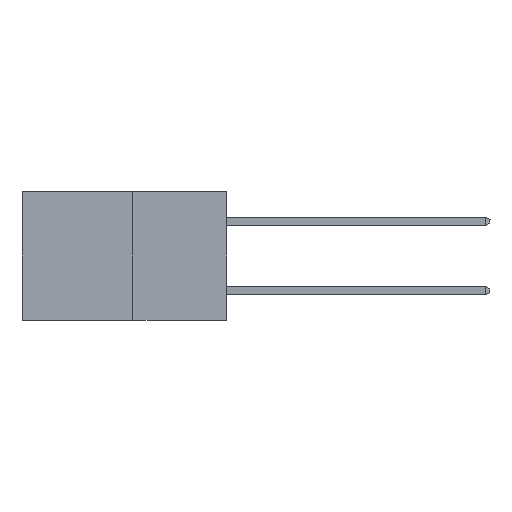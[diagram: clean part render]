
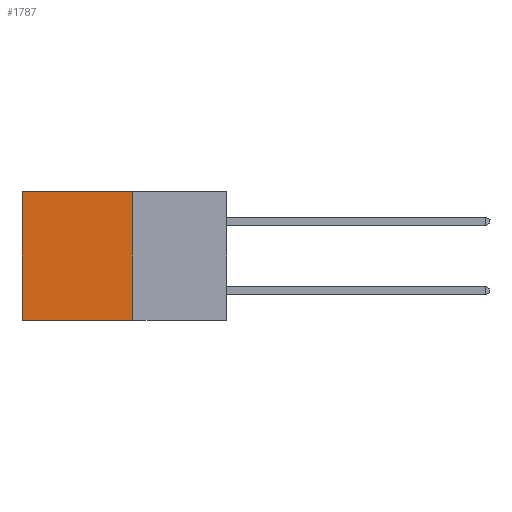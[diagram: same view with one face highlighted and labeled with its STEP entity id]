
A CAD part, left-side view. The second image highlights one B-rep face of the part: STEP entity #1787.
In plain terms, the highlighted planar face has unit normal (-1, 0, 0).
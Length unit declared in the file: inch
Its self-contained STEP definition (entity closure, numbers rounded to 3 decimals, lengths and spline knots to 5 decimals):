
#195 = VECTOR ( 'NONE', #348, 39.37008 ) ;
#211 = FACE_OUTER_BOUND ( 'NONE', #3395, .T. ) ;
#271 = DIRECTION ( 'NONE',  ( 0., 1., 0. ) ) ;
#348 = DIRECTION ( 'NONE',  ( 0., 0., -1. ) ) ;
#1368 = EDGE_CURVE ( 'NONE', #9910, #1708, #5854, .T. ) ;
#1708 = VERTEX_POINT ( 'NONE', #13616 ) ;
#1787 = ADVANCED_FACE ( 'NONE', ( #211 ), #13974, .F. ) ;
#1894 = CARTESIAN_POINT ( 'NONE',  ( 0.277, 0.27, -0.37 ) ) ;
#2162 = EDGE_CURVE ( 'NONE', #2884, #9910, #3405, .T. ) ;
#2731 = CARTESIAN_POINT ( 'NONE',  ( 0.277, 0.27, -0.37 ) ) ;
#2884 = VERTEX_POINT ( 'NONE', #9032 ) ;
#3395 = EDGE_LOOP ( 'NONE', ( #9013, #3718, #11988, #10713 ) ) ;
#3405 = LINE ( 'NONE', #1894, #195 ) ;
#3430 = EDGE_CURVE ( 'NONE', #4098, #1708, #4648, .T. ) ;
#3718 = ORIENTED_EDGE ( 'NONE', *, *, #1368, .F. ) ;
#3755 = CARTESIAN_POINT ( 'NONE',  ( 0.277, 0.59, -0.37 ) ) ;
#3772 = DIRECTION ( 'NONE',  ( 0., 0., -1. ) ) ;
#4098 = VERTEX_POINT ( 'NONE', #13778 ) ;
#4648 = LINE ( 'NONE', #3755, #13320 ) ;
#5483 = VECTOR ( 'NONE', #271, 39.37008 ) ;
#5854 = LINE ( 'NONE', #7898, #5483 ) ;
#6776 = DIRECTION ( 'NONE',  ( 0., 1., 0. ) ) ;
#6789 = CARTESIAN_POINT ( 'NONE',  ( 0.277, 0.27, 0. ) ) ;
#7898 = CARTESIAN_POINT ( 'NONE',  ( 0.277, 0.27, -0.37 ) ) ;
#9013 = ORIENTED_EDGE ( 'NONE', *, *, #3430, .T. ) ;
#9032 = CARTESIAN_POINT ( 'NONE',  ( 0.277, 0.27, 0. ) ) ;
#9784 = DIRECTION ( 'NONE',  ( 1., 0., 0. ) ) ;
#9819 = CARTESIAN_POINT ( 'NONE',  ( 0.277, 0.27, -0.37 ) ) ;
#9910 = VERTEX_POINT ( 'NONE', #2731 ) ;
#10713 = ORIENTED_EDGE ( 'NONE', *, *, #11121, .T. ) ;
#11121 = EDGE_CURVE ( 'NONE', #2884, #4098, #14993, .T. ) ;
#11988 = ORIENTED_EDGE ( 'NONE', *, *, #2162, .F. ) ;
#12680 = AXIS2_PLACEMENT_3D ( 'NONE', #9819, #9784, #13173 ) ;
#13173 = DIRECTION ( 'NONE',  ( 0., 0., -1. ) ) ;
#13320 = VECTOR ( 'NONE', #3772, 39.37008 ) ;
#13616 = CARTESIAN_POINT ( 'NONE',  ( 0.277, 0.59, -0.37 ) ) ;
#13778 = CARTESIAN_POINT ( 'NONE',  ( 0.277, 0.59, 0. ) ) ;
#13974 = PLANE ( 'NONE',  #12680 ) ;
#14674 = VECTOR ( 'NONE', #6776, 39.37008 ) ;
#14993 = LINE ( 'NONE', #6789, #14674 ) ;
